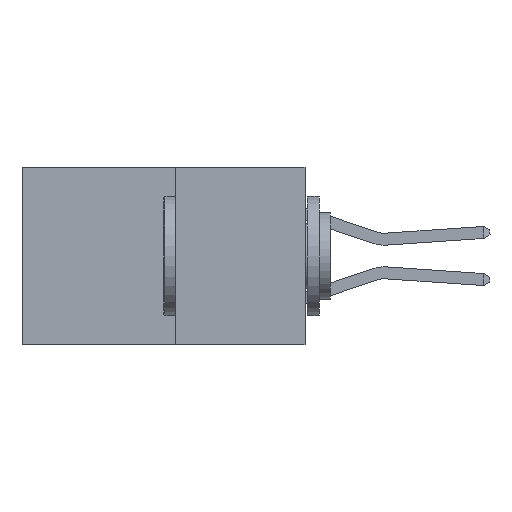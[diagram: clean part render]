
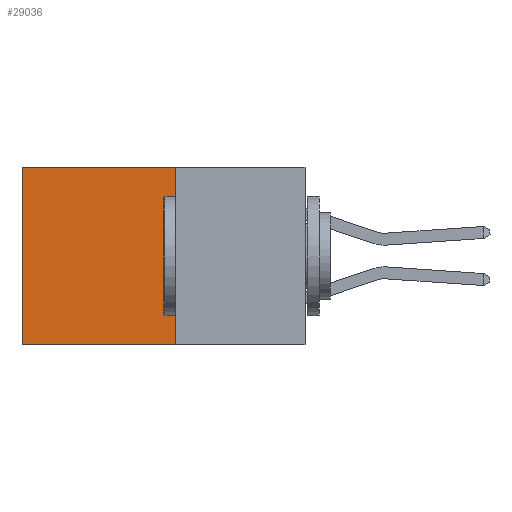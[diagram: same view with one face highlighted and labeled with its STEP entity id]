
A CAD part, left-side view. The second image highlights one B-rep face of the part: STEP entity #29036.
In plain terms, the highlighted planar face has unit normal (-1, 0, 0).
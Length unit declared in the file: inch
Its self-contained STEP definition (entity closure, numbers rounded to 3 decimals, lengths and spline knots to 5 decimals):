
#600 = VERTEX_POINT ( 'NONE', #7170 ) ;
#757 = EDGE_CURVE ( 'NONE', #600, #22044, #15370, .T. ) ;
#1445 = FACE_OUTER_BOUND ( 'NONE', #32554, .T. ) ;
#1595 = CARTESIAN_POINT ( 'NONE',  ( 0.277, 0.27, -0.37 ) ) ;
#3250 = ORIENTED_EDGE ( 'NONE', *, *, #757, .T. ) ;
#3333 = CARTESIAN_POINT ( 'NONE',  ( 0.277, 0.27, 0. ) ) ;
#4991 = AXIS2_PLACEMENT_3D ( 'NONE', #21125, #10050, #29437 ) ;
#6087 = CARTESIAN_POINT ( 'NONE',  ( 0.277, 0.27, -0.37 ) ) ;
#7170 = CARTESIAN_POINT ( 'NONE',  ( 0.277, 0.59, 0. ) ) ;
#10050 = DIRECTION ( 'NONE',  ( 1., 0., 0. ) ) ;
#10858 = VERTEX_POINT ( 'NONE', #6087 ) ;
#10884 = VERTEX_POINT ( 'NONE', #14450 ) ;
#12089 = VECTOR ( 'NONE', #22766, 39.37008 ) ;
#13102 = EDGE_CURVE ( 'NONE', #10884, #10858, #17968, .T. ) ;
#14450 = CARTESIAN_POINT ( 'NONE',  ( 0.277, 0.27, 0. ) ) ;
#15370 = LINE ( 'NONE', #33647, #21052 ) ;
#16636 = CARTESIAN_POINT ( 'NONE',  ( 0.277, 0.59, -0.37 ) ) ;
#17681 = VECTOR ( 'NONE', #24850, 39.37008 ) ;
#17968 = LINE ( 'NONE', #1595, #32662 ) ;
#19473 = LINE ( 'NONE', #3333, #12089 ) ;
#21040 = ORIENTED_EDGE ( 'NONE', *, *, #13102, .F. ) ;
#21052 = VECTOR ( 'NONE', #33699, 39.37008 ) ;
#21066 = DIRECTION ( 'NONE',  ( 0., 0., -1. ) ) ;
#21125 = CARTESIAN_POINT ( 'NONE',  ( 0.277, 0.27, -0.37 ) ) ;
#22044 = VERTEX_POINT ( 'NONE', #16636 ) ;
#22766 = DIRECTION ( 'NONE',  ( 0., 1., 0. ) ) ;
#23621 = ORIENTED_EDGE ( 'NONE', *, *, #26259, .F. ) ;
#24850 = DIRECTION ( 'NONE',  ( 0., 1., 0. ) ) ;
#25541 = ORIENTED_EDGE ( 'NONE', *, *, #26439, .T. ) ;
#26259 = EDGE_CURVE ( 'NONE', #10858, #22044, #32402, .T. ) ;
#26439 = EDGE_CURVE ( 'NONE', #10884, #600, #19473, .T. ) ;
#26669 = PLANE ( 'NONE',  #4991 ) ;
#27607 = CARTESIAN_POINT ( 'NONE',  ( 0.277, 0.27, -0.37 ) ) ;
#29036 = ADVANCED_FACE ( 'NONE', ( #1445 ), #26669, .F. ) ;
#29437 = DIRECTION ( 'NONE',  ( 0., 0., -1. ) ) ;
#32402 = LINE ( 'NONE', #27607, #17681 ) ;
#32554 = EDGE_LOOP ( 'NONE', ( #3250, #23621, #21040, #25541 ) ) ;
#32662 = VECTOR ( 'NONE', #21066, 39.37008 ) ;
#33647 = CARTESIAN_POINT ( 'NONE',  ( 0.277, 0.59, -0.37 ) ) ;
#33699 = DIRECTION ( 'NONE',  ( 0., 0., -1. ) ) ;
